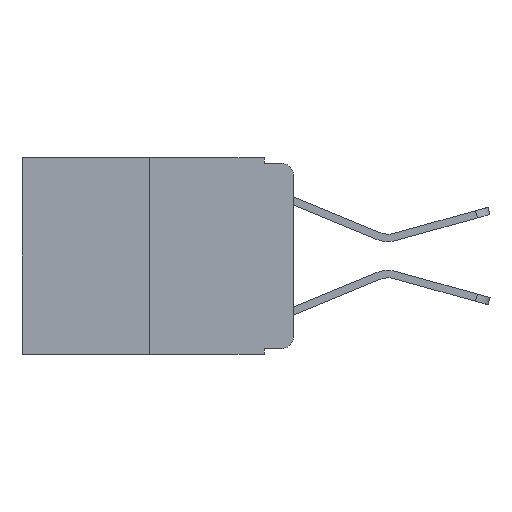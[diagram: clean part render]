
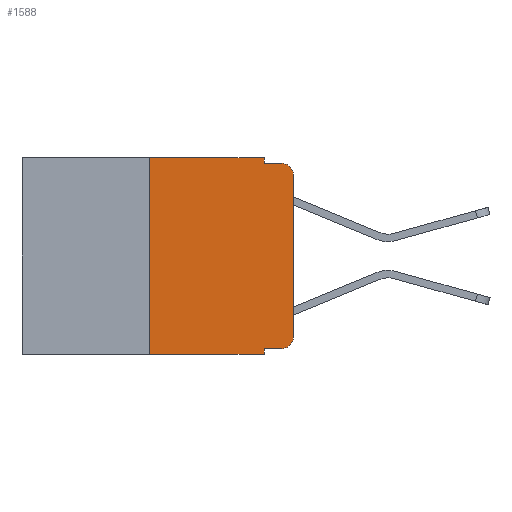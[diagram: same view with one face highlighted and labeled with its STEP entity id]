
A CAD part, left-side view. The second image highlights one B-rep face of the part: STEP entity #1588.
In plain terms, the highlighted planar face has unit normal (-1, 0, 0).
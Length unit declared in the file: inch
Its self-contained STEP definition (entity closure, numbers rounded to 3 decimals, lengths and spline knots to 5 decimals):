
#103 = VECTOR ( 'NONE', #9600, 39.37008 ) ;
#598 = DIRECTION ( 'NONE',  ( 0., -1., 0. ) ) ;
#679 = DIRECTION ( 'NONE',  ( -1., 0., 0. ) ) ;
#750 = CARTESIAN_POINT ( 'NONE',  ( 0., 0.051, -0.01 ) ) ;
#783 = EDGE_CURVE ( 'NONE', #15668, #11570, #10966, .T. ) ;
#908 = CARTESIAN_POINT ( 'NONE',  ( 0., 0.051, -0.333 ) ) ;
#958 = VERTEX_POINT ( 'NONE', #1174 ) ;
#1174 = CARTESIAN_POINT ( 'NONE',  ( 0., 0.051, -0.01 ) ) ;
#1588 = ADVANCED_FACE ( 'NONE', ( #15717 ), #3217, .F. ) ;
#1999 = DIRECTION ( 'NONE',  ( 0., 0., -1. ) ) ;
#2058 = CARTESIAN_POINT ( 'NONE',  ( 0., 0.473, 0. ) ) ;
#2069 = CARTESIAN_POINT ( 'NONE',  ( 0., 0.25, -0.343 ) ) ;
#3177 = CARTESIAN_POINT ( 'NONE',  ( 0., 0.473, 0. ) ) ;
#3217 = PLANE ( 'NONE',  #11069 ) ;
#3349 = ORIENTED_EDGE ( 'NONE', *, *, #7011, .F. ) ;
#3478 = VERTEX_POINT ( 'NONE', #3643 ) ;
#3571 = ORIENTED_EDGE ( 'NONE', *, *, #783, .T. ) ;
#3643 = CARTESIAN_POINT ( 'NONE',  ( 0., 0., -0.03 ) ) ;
#3727 = ORIENTED_EDGE ( 'NONE', *, *, #11593, .T. ) ;
#4050 = ORIENTED_EDGE ( 'NONE', *, *, #7149, .T. ) ;
#4299 = EDGE_CURVE ( 'NONE', #15860, #9592, #5774, .T. ) ;
#4382 = CARTESIAN_POINT ( 'NONE',  ( 0., 0.051, 0. ) ) ;
#4682 = EDGE_CURVE ( 'NONE', #9592, #958, #16797, .T. ) ;
#4718 = VECTOR ( 'NONE', #5602, 39.37008 ) ;
#4848 = LINE ( 'NONE', #13740, #12966 ) ;
#5032 = CARTESIAN_POINT ( 'NONE',  ( 0., 0.25, 0. ) ) ;
#5111 = EDGE_CURVE ( 'NONE', #3478, #8781, #11159, .T. ) ;
#5378 = ORIENTED_EDGE ( 'NONE', *, *, #6861, .F. ) ;
#5425 = DIRECTION ( 'NONE',  ( -1., 0., 0. ) ) ;
#5602 = DIRECTION ( 'NONE',  ( 0., 0., -1. ) ) ;
#5774 = LINE ( 'NONE', #3177, #8974 ) ;
#6354 = DIRECTION ( 'NONE',  ( 0., -1., 0. ) ) ;
#6485 = VECTOR ( 'NONE', #16156, 39.37008 ) ;
#6861 = EDGE_CURVE ( 'NONE', #13129, #15860, #4848, .T. ) ;
#6896 = ORIENTED_EDGE ( 'NONE', *, *, #4299, .F. ) ;
#7011 = EDGE_CURVE ( 'NONE', #958, #8781, #12779, .T. ) ;
#7149 = EDGE_CURVE ( 'NONE', #11570, #15331, #13168, .T. ) ;
#7462 = VECTOR ( 'NONE', #6354, 39.37008 ) ;
#7698 = AXIS2_PLACEMENT_3D ( 'NONE', #8787, #679, #15221 ) ;
#7944 = CARTESIAN_POINT ( 'NONE',  ( 0., 0.473, -0.343 ) ) ;
#8452 = DIRECTION ( 'NONE',  ( 0., 0., 1. ) ) ;
#8781 = VERTEX_POINT ( 'NONE', #12118 ) ;
#8787 = CARTESIAN_POINT ( 'NONE',  ( 0., 0.02, -0.03 ) ) ;
#8846 = ORIENTED_EDGE ( 'NONE', *, *, #5111, .T. ) ;
#8974 = VECTOR ( 'NONE', #598, 39.37008 ) ;
#9160 = CARTESIAN_POINT ( 'NONE',  ( 0., 0., -0.313 ) ) ;
#9323 = EDGE_CURVE ( 'NONE', #13129, #15697, #16199, .T. ) ;
#9592 = VERTEX_POINT ( 'NONE', #14954 ) ;
#9600 = DIRECTION ( 'NONE',  ( 0., 0., -1. ) ) ;
#10242 = EDGE_LOOP ( 'NONE', ( #3727, #8846, #3349, #13584, #6896, #5378, #10952, #14532, #3571, #4050 ) ) ;
#10778 = DIRECTION ( 'NONE',  ( 0., 0., -1. ) ) ;
#10847 = CARTESIAN_POINT ( 'NONE',  ( 0., 0.02, -0.333 ) ) ;
#10952 = ORIENTED_EDGE ( 'NONE', *, *, #9323, .T. ) ;
#10966 = LINE ( 'NONE', #908, #7462 ) ;
#11021 = CARTESIAN_POINT ( 'NONE',  ( 0., 0.051, 0. ) ) ;
#11069 = AXIS2_PLACEMENT_3D ( 'NONE', #2058, #13908, #1999 ) ;
#11094 = VECTOR ( 'NONE', #12668, 39.37008 ) ;
#11159 = CIRCLE ( 'NONE', #7698, 0.02 ) ;
#11570 = VERTEX_POINT ( 'NONE', #10847 ) ;
#11593 = EDGE_CURVE ( 'NONE', #15331, #3478, #15199, .T. ) ;
#11927 = DIRECTION ( 'NONE',  ( 0., -1., 0. ) ) ;
#12118 = CARTESIAN_POINT ( 'NONE',  ( 0., 0.02, -0.01 ) ) ;
#12668 = DIRECTION ( 'NONE',  ( 0., -1., 0. ) ) ;
#12779 = LINE ( 'NONE', #750, #11094 ) ;
#12912 = VECTOR ( 'NONE', #11927, 39.37008 ) ;
#12966 = VECTOR ( 'NONE', #8452, 39.37008 ) ;
#13129 = VERTEX_POINT ( 'NONE', #2069 ) ;
#13133 = AXIS2_PLACEMENT_3D ( 'NONE', #13388, #5425, #10778 ) ;
#13168 = CIRCLE ( 'NONE', #13133, 0.02 ) ;
#13388 = CARTESIAN_POINT ( 'NONE',  ( 0., 0.02, -0.313 ) ) ;
#13584 = ORIENTED_EDGE ( 'NONE', *, *, #4682, .F. ) ;
#13669 = CARTESIAN_POINT ( 'NONE',  ( 0., 0.051, -0.333 ) ) ;
#13740 = CARTESIAN_POINT ( 'NONE',  ( 0., 0.25, 0. ) ) ;
#13790 = LINE ( 'NONE', #4382, #103 ) ;
#13908 = DIRECTION ( 'NONE',  ( 1., 0., 0. ) ) ;
#14532 = ORIENTED_EDGE ( 'NONE', *, *, #16799, .F. ) ;
#14954 = CARTESIAN_POINT ( 'NONE',  ( 0., 0.051, 0. ) ) ;
#15199 = LINE ( 'NONE', #16220, #6485 ) ;
#15221 = DIRECTION ( 'NONE',  ( 0., 0., -1. ) ) ;
#15331 = VERTEX_POINT ( 'NONE', #9160 ) ;
#15668 = VERTEX_POINT ( 'NONE', #13669 ) ;
#15697 = VERTEX_POINT ( 'NONE', #16530 ) ;
#15717 = FACE_OUTER_BOUND ( 'NONE', #10242, .T. ) ;
#15860 = VERTEX_POINT ( 'NONE', #5032 ) ;
#16156 = DIRECTION ( 'NONE',  ( 0., 0., 1. ) ) ;
#16199 = LINE ( 'NONE', #7944, #12912 ) ;
#16220 = CARTESIAN_POINT ( 'NONE',  ( 0., 0., 0. ) ) ;
#16530 = CARTESIAN_POINT ( 'NONE',  ( 0., 0.051, -0.343 ) ) ;
#16797 = LINE ( 'NONE', #11021, #4718 ) ;
#16799 = EDGE_CURVE ( 'NONE', #15668, #15697, #13790, .T. ) ;
